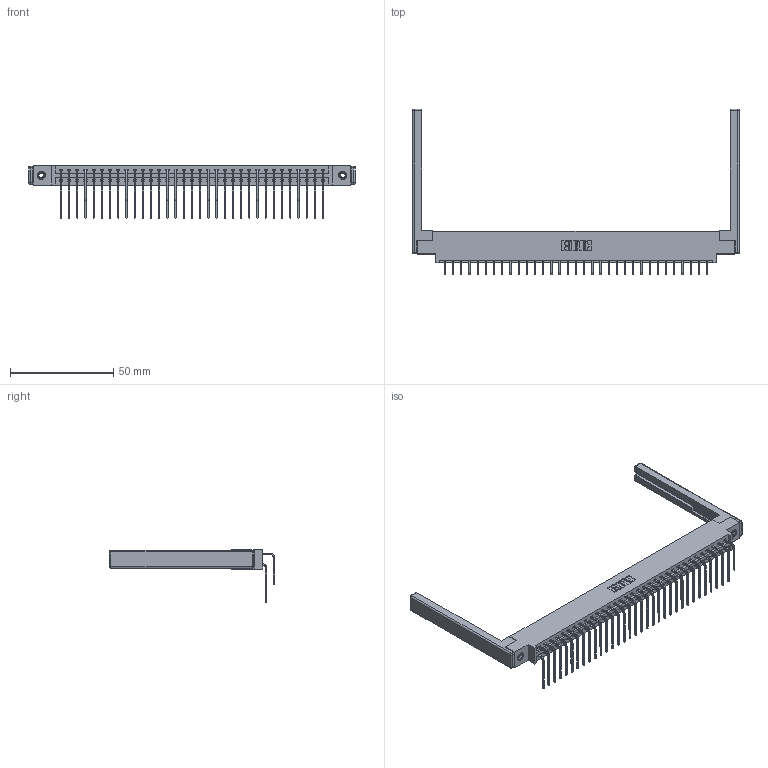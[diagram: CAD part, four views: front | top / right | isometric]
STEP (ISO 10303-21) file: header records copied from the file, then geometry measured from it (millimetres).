
FILE_DESCRIPTION (( 'STEP AP203' ), '1' );
FILE_NAME ('337-066-559-868.STEP', '2019-10-12T01:33:11', ( '' ), ( '' ), 'SwSTEP 2.0', 'SolidWorks 2016', '' );
FILE_SCHEMA (( 'CONFIG_CONTROL_DESIGN' ));
Length unit declared in the file: inch
Products named in the file (6): 337 Part_0.170 Offset - 0.156 Dia-TI; 345-292-001_558 559 Tail - 1; 345-292-001_559 Tail - 2; 307-220-068; 337-066-559-868; 345-250-001_345-250-001-102
Assembly tree (71 placements, depth 2):
  337-066-559-868
    337 Part_0.170 Offset - 0.156 Dia-TI
    345-292-001_558 559 Tail - 1  x33
    345-292-001_559 Tail - 2  x33
    345-250-001_345-250-001-102  x2
    307-220-068  x2
Bounding box: 158.19 x 79.95 x 25.53 mm (x, y, z)
Volume: 21199.7 mm3; surface area: 24975.8 mm2
Topology: 71 solids, 71 shells, 3968 faces, 11735 edges, 7714 vertices
Faces by surface type: plane 2802, cylinder 1142, cone 12, sphere 8, torus 4
Entity records: 31426 total; most frequent: CARTESIAN_POINT 5314, ORIENTED_EDGE 5188, DIRECTION 4588, EDGE_CURVE 2594, LINE 2376, VECTOR 2376, VERTEX_POINT 1718, AXIS2_PLACEMENT_3D 1106
